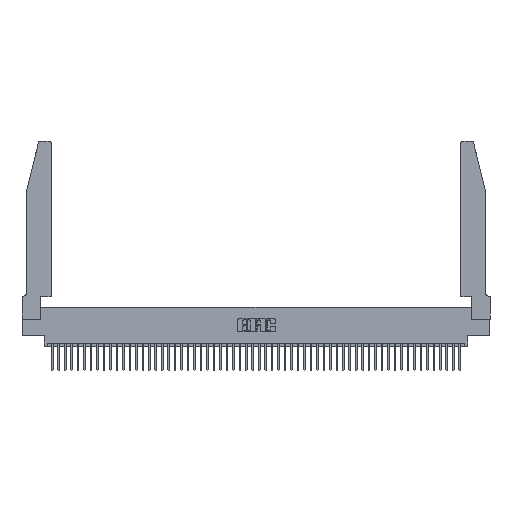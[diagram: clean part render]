
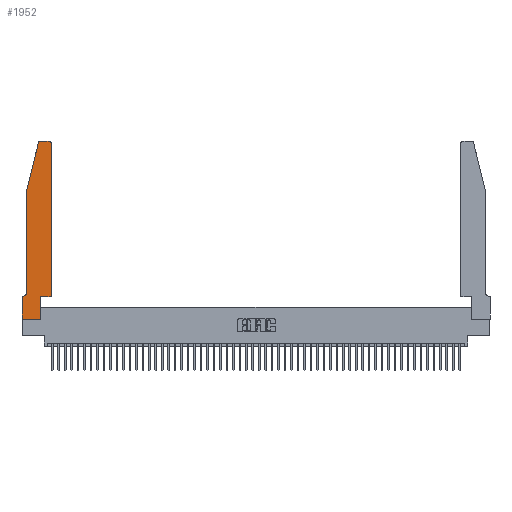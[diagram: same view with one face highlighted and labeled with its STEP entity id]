
A CAD part, top view. The second image highlights one B-rep face of the part: STEP entity #1952.
In plain terms, the highlighted planar face has unit normal (0, 0, 1).
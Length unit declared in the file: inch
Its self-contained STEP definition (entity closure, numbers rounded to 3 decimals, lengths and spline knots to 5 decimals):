
#185 = EDGE_CURVE ( 'NONE', #24361, #11561, #8331, .T. ) ;
#1113 = LINE ( 'NONE', #17558, #10589 ) ;
#1519 = ORIENTED_EDGE ( 'NONE', *, *, #45426, .T. ) ;
#1597 = CARTESIAN_POINT ( 'NONE',  ( 0.2605, 2.75, 0.37 ) ) ;
#1943 = LINE ( 'NONE', #45493, #11435 ) ;
#1952 = ADVANCED_FACE ( 'NONE', ( #6958 ), #26810, .T. ) ;
#1996 = LINE ( 'NONE', #6272, #43621 ) ;
#2301 = CARTESIAN_POINT ( 'NONE',  ( 0.4205, 2.75, 0.37 ) ) ;
#2406 = CARTESIAN_POINT ( 'NONE',  ( 0., 0., 0.37 ) ) ;
#2945 = EDGE_CURVE ( 'NONE', #47108, #12214, #22886, .T. ) ;
#3433 = EDGE_CURVE ( 'NONE', #47860, #25441, #22839, .T. ) ;
#3725 = EDGE_CURVE ( 'NONE', #25363, #20855, #19659, .T. ) ;
#4252 = ORIENTED_EDGE ( 'NONE', *, *, #44358, .T. ) ;
#4600 = CARTESIAN_POINT ( 'NONE',  ( 0.4505, 0.35, 0.37 ) ) ;
#4932 = DIRECTION ( 'NONE',  ( 0., -1., 0. ) ) ;
#5551 = CARTESIAN_POINT ( 'NONE',  ( 0.4205, 2.72, 0.37 ) ) ;
#5770 = CARTESIAN_POINT ( 'NONE',  ( 0.0755, 0.42, 0.37 ) ) ;
#5976 = CARTESIAN_POINT ( 'NONE',  ( 0.284, 2.75, 0.37 ) ) ;
#6272 = CARTESIAN_POINT ( 'NONE',  ( 0.2865, 0.35, 0.37 ) ) ;
#6567 = ORIENTED_EDGE ( 'NONE', *, *, #3725, .T. ) ;
#6622 = ORIENTED_EDGE ( 'NONE', *, *, #50062, .T. ) ;
#6709 = DIRECTION ( 'NONE',  ( 1., 0., 0. ) ) ;
#6958 = FACE_OUTER_BOUND ( 'NONE', #12681, .T. ) ;
#7201 = VECTOR ( 'NONE', #15709, 39.37008 ) ;
#8331 = LINE ( 'NONE', #10986, #51144 ) ;
#8893 = CARTESIAN_POINT ( 'NONE',  ( 0.2865, 0., 0.37 ) ) ;
#8991 = CARTESIAN_POINT ( 'NONE',  ( 0., 0., 0.37 ) ) ;
#9600 = DIRECTION ( 'NONE',  ( 1., 0., 0. ) ) ;
#9990 = EDGE_CURVE ( 'NONE', #34358, #24361, #33386, .T. ) ;
#10589 = VECTOR ( 'NONE', #49737, 39.37008 ) ;
#10986 = CARTESIAN_POINT ( 'NONE',  ( 0., 0., 0.37 ) ) ;
#11435 = VECTOR ( 'NONE', #17350, 39.37008 ) ;
#11561 = VERTEX_POINT ( 'NONE', #8893 ) ;
#12214 = VERTEX_POINT ( 'NONE', #4600 ) ;
#12418 = CARTESIAN_POINT ( 'NONE',  ( 0.284, 2.72, 0.37 ) ) ;
#12681 = EDGE_LOOP ( 'NONE', ( #6622, #50720, #51885, #6567, #1519, #41348, #23639, #31908, #4252, #36126, #19404, #13611 ) ) ;
#12891 = CARTESIAN_POINT ( 'NONE',  ( 0.0055, 0.42, 0.37 ) ) ;
#13317 = AXIS2_PLACEMENT_3D ( 'NONE', #5551, #33741, #9600 ) ;
#13524 = CARTESIAN_POINT ( 'NONE',  ( 0.4505, 0.35, 0.37 ) ) ;
#13611 = ORIENTED_EDGE ( 'NONE', *, *, #31693, .T. ) ;
#13992 = DIRECTION ( 'NONE',  ( 0., -1., 0. ) ) ;
#15709 = DIRECTION ( 'NONE',  ( 0., 1., 0. ) ) ;
#16480 = DIRECTION ( 'NONE',  ( 1., 0., 0. ) ) ;
#16944 = DIRECTION ( 'NONE',  ( -1., 0., 0. ) ) ;
#17061 = CIRCLE ( 'NONE', #24479, 0.07 ) ;
#17350 = DIRECTION ( 'NONE',  ( -1., 0., 0. ) ) ;
#17558 = CARTESIAN_POINT ( 'NONE',  ( 0.0755, 2., 0.37 ) ) ;
#17966 = VERTEX_POINT ( 'NONE', #20874 ) ;
#18646 = CARTESIAN_POINT ( 'NONE',  ( 0.25487, 2.72718, 0.37 ) ) ;
#19404 = ORIENTED_EDGE ( 'NONE', *, *, #42227, .T. ) ;
#19659 = LINE ( 'NONE', #34201, #20929 ) ;
#20855 = VERTEX_POINT ( 'NONE', #5770 ) ;
#20874 = CARTESIAN_POINT ( 'NONE',  ( 0.0055, 0.35, 0.37 ) ) ;
#20929 = VECTOR ( 'NONE', #13992, 39.37008 ) ;
#21389 = AXIS2_PLACEMENT_3D ( 'NONE', #12418, #40599, #16480 ) ;
#21918 = CARTESIAN_POINT ( 'NONE',  ( 0.2865, 0.35, 0.37 ) ) ;
#22773 = CARTESIAN_POINT ( 'NONE',  ( 0., 0.35, 0.37 ) ) ;
#22839 = CIRCLE ( 'NONE', #21389, 0.03 ) ;
#22886 = LINE ( 'NONE', #13524, #33587 ) ;
#23639 = ORIENTED_EDGE ( 'NONE', *, *, #9990, .T. ) ;
#24361 = VERTEX_POINT ( 'NONE', #2406 ) ;
#24479 = AXIS2_PLACEMENT_3D ( 'NONE', #12891, #41067, #16944 ) ;
#25363 = VERTEX_POINT ( 'NONE', #41954 ) ;
#25441 = VERTEX_POINT ( 'NONE', #18646 ) ;
#26810 = PLANE ( 'NONE',  #36190 ) ;
#26903 = VECTOR ( 'NONE', #29786, 39.37008 ) ;
#29786 = DIRECTION ( 'NONE',  ( -1., 0., 0. ) ) ;
#30396 = DIRECTION ( 'NONE',  ( 0., 1., 0. ) ) ;
#30831 = DIRECTION ( 'NONE',  ( 0., 0., 1. ) ) ;
#31693 = EDGE_CURVE ( 'NONE', #45482, #32453, #41437, .T. ) ;
#31908 = ORIENTED_EDGE ( 'NONE', *, *, #185, .T. ) ;
#32453 = VERTEX_POINT ( 'NONE', #2301 ) ;
#33136 = CARTESIAN_POINT ( 'NONE',  ( 0.4505, 2.72, 0.37 ) ) ;
#33386 = LINE ( 'NONE', #8991, #42827 ) ;
#33583 = DIRECTION ( 'NONE',  ( 1., 0., 0. ) ) ;
#33587 = VECTOR ( 'NONE', #33583, 39.37008 ) ;
#33741 = DIRECTION ( 'NONE',  ( 0., 0., 1. ) ) ;
#34201 = CARTESIAN_POINT ( 'NONE',  ( 0.0755, 2., 0.37 ) ) ;
#34358 = VERTEX_POINT ( 'NONE', #22773 ) ;
#34712 = CARTESIAN_POINT ( 'NONE',  ( 0., 0.35, 0.37 ) ) ;
#35106 = DIRECTION ( 'NONE',  ( 1., 0., 0. ) ) ;
#35758 = CARTESIAN_POINT ( 'NONE',  ( 0.4505, 0.35, 0.37 ) ) ;
#36126 = ORIENTED_EDGE ( 'NONE', *, *, #2945, .T. ) ;
#36190 = AXIS2_PLACEMENT_3D ( 'NONE', #34712, #30831, #6709 ) ;
#37607 = LINE ( 'NONE', #1597, #26903 ) ;
#40599 = DIRECTION ( 'NONE',  ( 0., 0., 1. ) ) ;
#41067 = DIRECTION ( 'NONE',  ( 0., 0., -1. ) ) ;
#41348 = ORIENTED_EDGE ( 'NONE', *, *, #44875, .T. ) ;
#41437 = CIRCLE ( 'NONE', #13317, 0.03 ) ;
#41954 = CARTESIAN_POINT ( 'NONE',  ( 0.0755, 2., 0.37 ) ) ;
#42227 = EDGE_CURVE ( 'NONE', #12214, #45482, #47523, .T. ) ;
#42827 = VECTOR ( 'NONE', #4932, 39.37008 ) ;
#43621 = VECTOR ( 'NONE', #30396, 39.37008 ) ;
#44358 = EDGE_CURVE ( 'NONE', #11561, #47108, #1996, .T. ) ;
#44875 = EDGE_CURVE ( 'NONE', #17966, #34358, #1943, .T. ) ;
#45426 = EDGE_CURVE ( 'NONE', #20855, #17966, #17061, .T. ) ;
#45482 = VERTEX_POINT ( 'NONE', #33136 ) ;
#45493 = CARTESIAN_POINT ( 'NONE',  ( 0.0755, 0.35, 0.37 ) ) ;
#47108 = VERTEX_POINT ( 'NONE', #21918 ) ;
#47523 = LINE ( 'NONE', #35758, #7201 ) ;
#47860 = VERTEX_POINT ( 'NONE', #5976 ) ;
#48437 = EDGE_CURVE ( 'NONE', #25441, #25363, #1113, .T. ) ;
#49737 = DIRECTION ( 'NONE',  ( -0.239, -0.971, 0. ) ) ;
#50062 = EDGE_CURVE ( 'NONE', #32453, #47860, #37607, .T. ) ;
#50720 = ORIENTED_EDGE ( 'NONE', *, *, #3433, .T. ) ;
#51144 = VECTOR ( 'NONE', #35106, 39.37008 ) ;
#51885 = ORIENTED_EDGE ( 'NONE', *, *, #48437, .T. ) ;
